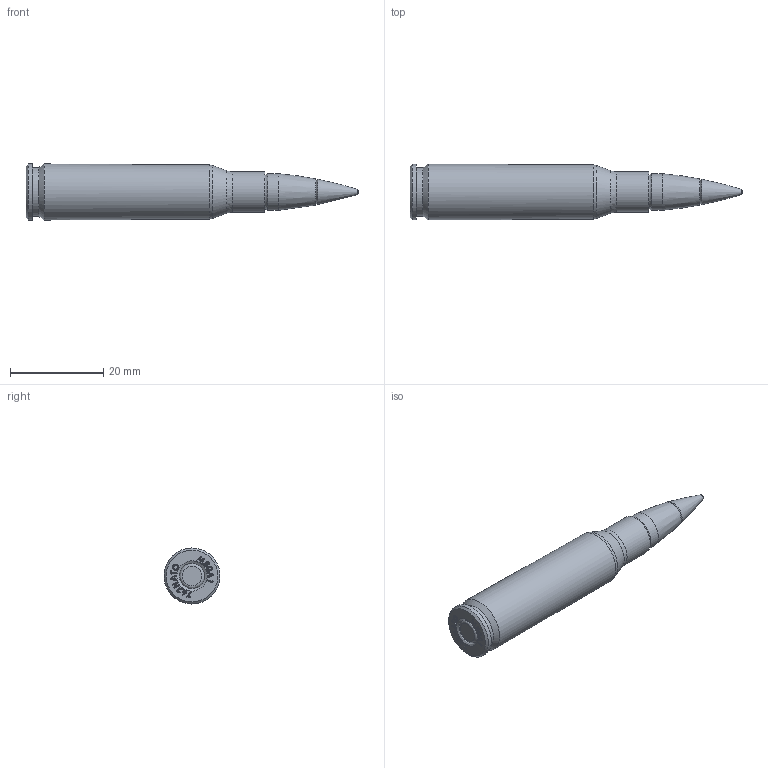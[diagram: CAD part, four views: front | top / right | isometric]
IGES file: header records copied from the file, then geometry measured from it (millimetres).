
Global section: file name: .308 win NATO M80A1; native system: Autodesk Inventor 2021; preprocessor: unknown; author: user; date: 20201230.053628; units: millimetre
Bounding box: 71.12 x 11.99 x 12.01 mm (x, y, z)
Volume: 2543.9 mm3; surface area: 5490.2 mm2
Topology: 7 solids, 7 shells, 357 faces, 853 edges, 532 vertices
Faces by surface type: bspline 357
